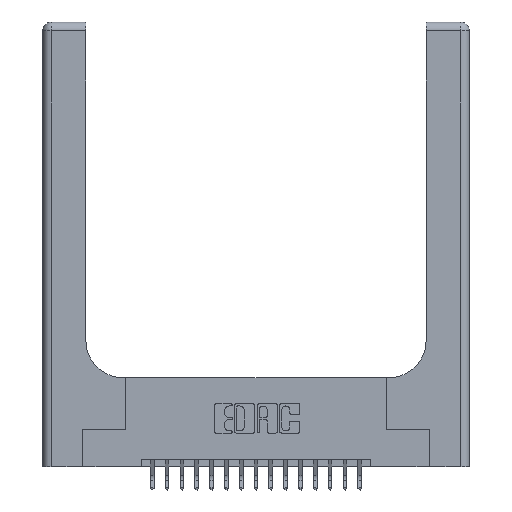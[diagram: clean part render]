
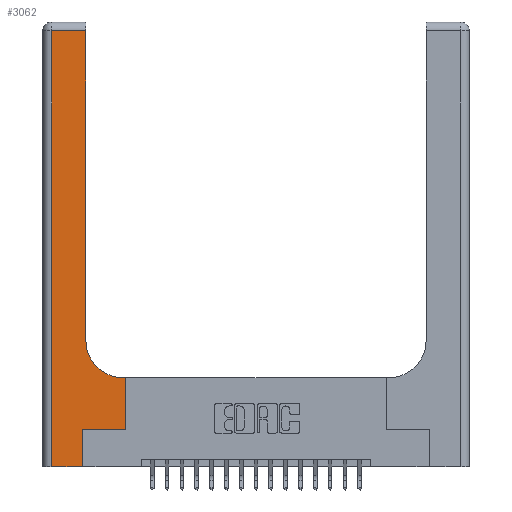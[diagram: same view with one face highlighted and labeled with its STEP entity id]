
A CAD part, top view. The second image highlights one B-rep face of the part: STEP entity #3062.
In plain terms, the highlighted planar face has unit normal (0, 0, 1).
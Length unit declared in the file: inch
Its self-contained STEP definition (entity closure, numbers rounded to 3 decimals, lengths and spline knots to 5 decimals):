
#200 = EDGE_LOOP ( 'NONE', ( #20014, #20484, #14002, #18076, #1837, #16743, #18330, #15769, #14792 ) ) ;
#795 = CARTESIAN_POINT ( 'NONE',  ( 0., 3., 0.37 ) ) ;
#1025 = VECTOR ( 'NONE', #12405, 39.37008 ) ;
#1246 = EDGE_CURVE ( 'NONE', #4733, #1869, #9506, .T. ) ;
#1548 = DIRECTION ( 'NONE',  ( -1., 0., 0. ) ) ;
#1837 = ORIENTED_EDGE ( 'NONE', *, *, #4571, .T. ) ;
#1869 = VERTEX_POINT ( 'NONE', #13795 ) ;
#2552 = LINE ( 'NONE', #12269, #9869 ) ;
#2565 = DIRECTION ( 'NONE',  ( 0., 0., -1. ) ) ;
#2975 = DIRECTION ( 'NONE',  ( 0., 1., 0. ) ) ;
#3062 = ADVANCED_FACE ( 'NONE', ( #5593 ), #12197, .F. ) ;
#3150 = EDGE_CURVE ( 'NONE', #13621, #20620, #12399, .T. ) ;
#3301 = CARTESIAN_POINT ( 'NONE',  ( 0.269, 0., 0.37 ) ) ;
#3509 = VECTOR ( 'NONE', #2975, 39.37008 ) ;
#3589 = EDGE_CURVE ( 'NONE', #10992, #17031, #20450, .T. ) ;
#4078 = DIRECTION ( 'NONE',  ( 1., 0., 0. ) ) ;
#4234 = CARTESIAN_POINT ( 'NONE',  ( 0.5415, 0.6, 0.37 ) ) ;
#4344 = DIRECTION ( 'NONE',  ( 0., 0., -1. ) ) ;
#4571 = EDGE_CURVE ( 'NONE', #7949, #10992, #18939, .T. ) ;
#4733 = VERTEX_POINT ( 'NONE', #15147 ) ;
#4852 = EDGE_CURVE ( 'NONE', #10188, #4733, #9615, .T. ) ;
#5593 = FACE_OUTER_BOUND ( 'NONE', #200, .T. ) ;
#6150 = CARTESIAN_POINT ( 'NONE',  ( 0.2915, 0.85, 0.37 ) ) ;
#6187 = CARTESIAN_POINT ( 'NONE',  ( 0.2915, 2.94, 0.37 ) ) ;
#6239 = VERTEX_POINT ( 'NONE', #18419 ) ;
#6322 = CARTESIAN_POINT ( 'NONE',  ( 0.2915, 0.6, 0.37 ) ) ;
#6435 = LINE ( 'NONE', #6322, #10179 ) ;
#6533 = DIRECTION ( 'NONE',  ( 0., 1., 0. ) ) ;
#6611 = AXIS2_PLACEMENT_3D ( 'NONE', #18903, #4344, #15591 ) ;
#6852 = LINE ( 'NONE', #11618, #7609 ) ;
#7609 = VECTOR ( 'NONE', #19515, 39.37008 ) ;
#7693 = AXIS2_PLACEMENT_3D ( 'NONE', #795, #2565, #13825 ) ;
#7949 = VERTEX_POINT ( 'NONE', #9045 ) ;
#8943 = CARTESIAN_POINT ( 'NONE',  ( 0.269, 0.25, 0.37 ) ) ;
#9045 = CARTESIAN_POINT ( 'NONE',  ( 0.269, 0., 0.37 ) ) ;
#9121 = DIRECTION ( 'NONE',  ( 0., -1., 0. ) ) ;
#9182 = EDGE_CURVE ( 'NONE', #1869, #7949, #6852, .T. ) ;
#9506 = LINE ( 'NONE', #18743, #12238 ) ;
#9615 = LINE ( 'NONE', #17197, #1025 ) ;
#9869 = VECTOR ( 'NONE', #20346, 39.37008 ) ;
#10179 = VECTOR ( 'NONE', #1548, 39.37008 ) ;
#10188 = VERTEX_POINT ( 'NONE', #6187 ) ;
#10814 = EDGE_CURVE ( 'NONE', #17031, #6239, #17086, .T. ) ;
#10879 = VECTOR ( 'NONE', #4078, 39.37008 ) ;
#10992 = VERTEX_POINT ( 'NONE', #19952 ) ;
#11122 = CARTESIAN_POINT ( 'NONE',  ( 0.5585, 0.25, 0.37 ) ) ;
#11618 = CARTESIAN_POINT ( 'NONE',  ( 0., 0., 0.37 ) ) ;
#12197 = PLANE ( 'NONE',  #7693 ) ;
#12238 = VECTOR ( 'NONE', #9121, 39.37008 ) ;
#12269 = CARTESIAN_POINT ( 'NONE',  ( 0.2915, 3., 0.37 ) ) ;
#12399 = CIRCLE ( 'NONE', #6611, 0.25 ) ;
#12405 = DIRECTION ( 'NONE',  ( -1., 0., 0. ) ) ;
#13621 = VERTEX_POINT ( 'NONE', #4234 ) ;
#13795 = CARTESIAN_POINT ( 'NONE',  ( 0.06, 0., 0.37 ) ) ;
#13825 = DIRECTION ( 'NONE',  ( -1., 0., 0. ) ) ;
#14002 = ORIENTED_EDGE ( 'NONE', *, *, #1246, .T. ) ;
#14643 = VECTOR ( 'NONE', #6533, 39.37008 ) ;
#14792 = ORIENTED_EDGE ( 'NONE', *, *, #3150, .T. ) ;
#15147 = CARTESIAN_POINT ( 'NONE',  ( 0.06, 2.94, 0.37 ) ) ;
#15271 = EDGE_CURVE ( 'NONE', #20620, #10188, #2552, .T. ) ;
#15591 = DIRECTION ( 'NONE',  ( 1., 0., 0. ) ) ;
#15769 = ORIENTED_EDGE ( 'NONE', *, *, #20193, .T. ) ;
#16743 = ORIENTED_EDGE ( 'NONE', *, *, #3589, .T. ) ;
#17031 = VERTEX_POINT ( 'NONE', #19969 ) ;
#17086 = LINE ( 'NONE', #11122, #3509 ) ;
#17197 = CARTESIAN_POINT ( 'NONE',  ( 0., 2.94, 0.37 ) ) ;
#18076 = ORIENTED_EDGE ( 'NONE', *, *, #9182, .T. ) ;
#18330 = ORIENTED_EDGE ( 'NONE', *, *, #10814, .T. ) ;
#18419 = CARTESIAN_POINT ( 'NONE',  ( 0.5585, 0.6, 0.37 ) ) ;
#18743 = CARTESIAN_POINT ( 'NONE',  ( 0.06, 3., 0.37 ) ) ;
#18903 = CARTESIAN_POINT ( 'NONE',  ( 0.5415, 0.85, 0.37 ) ) ;
#18939 = LINE ( 'NONE', #3301, #14643 ) ;
#19515 = DIRECTION ( 'NONE',  ( 1., 0., 0. ) ) ;
#19952 = CARTESIAN_POINT ( 'NONE',  ( 0.269, 0.25, 0.37 ) ) ;
#19969 = CARTESIAN_POINT ( 'NONE',  ( 0.5585, 0.25, 0.37 ) ) ;
#20014 = ORIENTED_EDGE ( 'NONE', *, *, #15271, .T. ) ;
#20193 = EDGE_CURVE ( 'NONE', #6239, #13621, #6435, .T. ) ;
#20346 = DIRECTION ( 'NONE',  ( 0., 1., 0. ) ) ;
#20450 = LINE ( 'NONE', #8943, #10879 ) ;
#20484 = ORIENTED_EDGE ( 'NONE', *, *, #4852, .T. ) ;
#20620 = VERTEX_POINT ( 'NONE', #6150 ) ;
